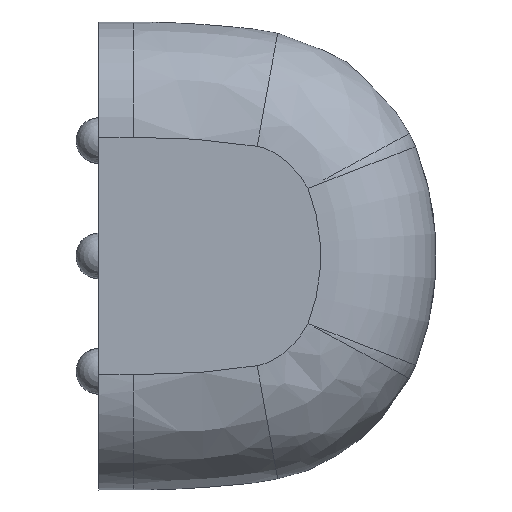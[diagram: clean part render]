
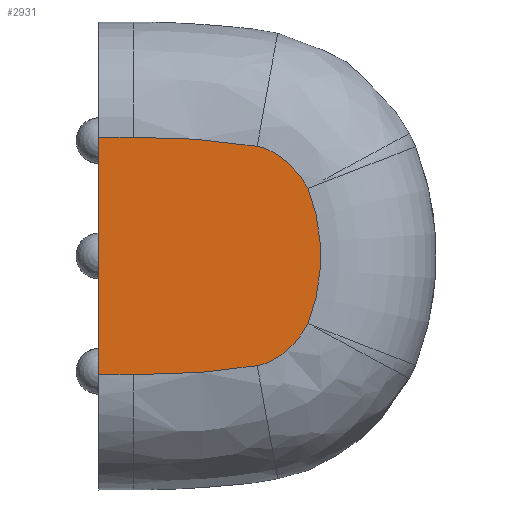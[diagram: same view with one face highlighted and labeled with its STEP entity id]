
A CAD part, front view. The second image highlights one B-rep face of the part: STEP entity #2931.
In plain terms, the highlighted planar face has unit normal (0, -1, 0).
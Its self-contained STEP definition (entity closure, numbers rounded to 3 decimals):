
#60 = PLANE ( 'NONE',  #2061 ) ;
#94 = LINE ( 'NONE', #3117, #1246 ) ;
#139 = ORIENTED_EDGE ( 'NONE', *, *, #1012, .T. ) ;
#150 = CARTESIAN_POINT ( 'NONE',  ( -197.151, -79.943, -4.872 ) ) ;
#158 = CARTESIAN_POINT ( 'NONE',  ( -194.189, -79.943, 11.849 ) ) ;
#170 = VECTOR ( 'NONE', #3133, 1000. ) ;
#292 = ORIENTED_EDGE ( 'NONE', *, *, #4550, .T. ) ;
#363 = EDGE_CURVE ( 'NONE', #2979, #3120, #4912, .T. ) ;
#495 = VERTEX_POINT ( 'NONE', #5963 ) ;
#546 = B_SPLINE_CURVE_WITH_KNOTS ( 'NONE', 3,
 ( #2611, #150, #666, #4102, #1153, #4589, #1658, #5085, #2151, #5576, #2631, #6057 ),
 .UNSPECIFIED., .F., .F.,
 ( 4, 2, 2, 2, 2, 4 ),
 ( 0., 0.001, 0.002, 0.003, 0.004, 0.006 ),
 .UNSPECIFIED. ) ;
#556 = CARTESIAN_POINT ( 'NONE',  ( -193.644, -79.943, -21.728 ) ) ;
#651 = CARTESIAN_POINT ( 'NONE',  ( -194.688, -79.943, 12.395 ) ) ;
#666 = CARTESIAN_POINT ( 'NONE',  ( -196.694, -79.943, -4.699 ) ) ;
#692 = EDGE_CURVE ( 'NONE', #1671, #495, #546, .T. ) ;
#695 = CARTESIAN_POINT ( 'NONE',  ( -201.21, -79.943, 14.543 ) ) ;
#735 = ORIENTED_EDGE ( 'NONE', *, *, #5508, .T. ) ;
#886 = CARTESIAN_POINT ( 'NONE',  ( -202.107, -79.943, -5.524 ) ) ;
#904 = VERTEX_POINT ( 'NONE', #3021 ) ;
#1001 = FACE_OUTER_BOUND ( 'NONE', #3509, .T. ) ;
#1012 = EDGE_CURVE ( 'NONE', #904, #1671, #2285, .T. ) ;
#1022 = AXIS2_PLACEMENT_3D ( 'NONE', #2161, #5590, #2644 ) ;
#1037 = DIRECTION ( 'NONE',  ( 0., 0., -1. ) ) ;
#1045 = DIRECTION ( 'NONE',  ( 0., 1., 0. ) ) ;
#1140 = CARTESIAN_POINT ( 'NONE',  ( -195.233, -79.943, 12.886 ) ) ;
#1153 = CARTESIAN_POINT ( 'NONE',  ( -195.832, -79.943, -4.226 ) ) ;
#1186 = CARTESIAN_POINT ( 'NONE',  ( -204.803, -79.943, 14.792 ) ) ;
#1246 = VECTOR ( 'NONE', #5556, 1000. ) ;
#1385 = CARTESIAN_POINT ( 'NONE',  ( -199.42, -79.943, -5.248 ) ) ;
#1530 = ORIENTED_EDGE ( 'NONE', *, *, #2436, .T. ) ;
#1644 = CARTESIAN_POINT ( 'NONE',  ( -195.828, -79.943, 13.318 ) ) ;
#1658 = CARTESIAN_POINT ( 'NONE',  ( -195.233, -79.943, -3.792 ) ) ;
#1671 = VERTEX_POINT ( 'NONE', #2897 ) ;
#1691 = CARTESIAN_POINT ( 'NONE',  ( -208.404, -79.943, 14.84 ) ) ;
#1882 = CARTESIAN_POINT ( 'NONE',  ( -197.642, -79.943, -4.962 ) ) ;
#1894 = CARTESIAN_POINT ( 'NONE',  ( -211.361, -79.943, -5.745 ) ) ;
#1913 = VERTEX_POINT ( 'NONE', #3108 ) ;
#1935 = EDGE_CURVE ( 'NONE', #4281, #904, #2935, .T. ) ;
#2061 = AXIS2_PLACEMENT_3D ( 'NONE', #556, #1045, #4484 ) ;
#2136 = CARTESIAN_POINT ( 'NONE',  ( -196.694, -79.943, 13.794 ) ) ;
#2151 = CARTESIAN_POINT ( 'NONE',  ( -194.346, -79.943, -2.954 ) ) ;
#2161 = CARTESIAN_POINT ( 'NONE',  ( -208.404, -79.943, 4.547 ) ) ;
#2285 = B_SPLINE_CURVE_WITH_KNOTS ( 'NONE', 3,
 ( #2358, #5292, #3830, #886, #4326, #1385, #4818, #1882 ),
 .UNSPECIFIED., .F., .F.,
 ( 4, 2, 2, 4 ),
 ( 0., 0.005, 0.008, 0.011 ),
 .UNSPECIFIED. ) ;
#2358 = CARTESIAN_POINT ( 'NONE',  ( -208.403, -79.943, -5.745 ) ) ;
#2436 = EDGE_CURVE ( 'NONE', #5596, #1913, #94, .T. ) ;
#2483 = CARTESIAN_POINT ( 'NONE',  ( -211.361, -79.943, -21.728 ) ) ;
#2600 = CARTESIAN_POINT ( 'NONE',  ( -193.466, -79.943, 10.854 ) ) ;
#2611 = CARTESIAN_POINT ( 'NONE',  ( -197.642, -79.943, -4.962 ) ) ;
#2619 = CARTESIAN_POINT ( 'NONE',  ( -197.642, -79.943, 14.056 ) ) ;
#2631 = CARTESIAN_POINT ( 'NONE',  ( -193.466, -79.943, -1.759 ) ) ;
#2642 = CARTESIAN_POINT ( 'NONE',  ( -197.642, -79.943, 14.056 ) ) ;
#2644 = DIRECTION ( 'NONE',  ( -1., 0., 0. ) ) ;
#2897 = CARTESIAN_POINT ( 'NONE',  ( -197.642, -79.943, -4.962 ) ) ;
#2931 = ADVANCED_FACE ( 'NONE', ( #1001 ), #60, .F. ) ;
#2935 = LINE ( 'NONE', #5571, #170 ) ;
#2979 = VERTEX_POINT ( 'NONE', #4503 ) ;
#3021 = CARTESIAN_POINT ( 'NONE',  ( -208.403, -79.943, -5.745 ) ) ;
#3108 = CARTESIAN_POINT ( 'NONE',  ( -211.361, -79.943, 14.84 ) ) ;
#3117 = CARTESIAN_POINT ( 'NONE',  ( -193.644, -79.943, 14.84 ) ) ;
#3120 = VERTEX_POINT ( 'NONE', #4561 ) ;
#3133 = DIRECTION ( 'NONE',  ( 1., 0., 0. ) ) ;
#3509 = EDGE_LOOP ( 'NONE', ( #1530, #735, #3752, #139, #5740, #292, #4438, #4811 ) ) ;
#3585 = CIRCLE ( 'NONE', #1022, 16.269 ) ;
#3605 = CARTESIAN_POINT ( 'NONE',  ( -194.35, -79.943, 12.037 ) ) ;
#3642 = CARTESIAN_POINT ( 'NONE',  ( -199.42, -79.943, 14.342 ) ) ;
#3752 = ORIENTED_EDGE ( 'NONE', *, *, #1935, .T. ) ;
#3830 = CARTESIAN_POINT ( 'NONE',  ( -204.803, -79.943, -5.697 ) ) ;
#4090 = CARTESIAN_POINT ( 'NONE',  ( -194.864, -79.943, 12.565 ) ) ;
#4102 = CARTESIAN_POINT ( 'NONE',  ( -196.044, -79.943, -4.356 ) ) ;
#4134 = CARTESIAN_POINT ( 'NONE',  ( -202.107, -79.943, 14.618 ) ) ;
#4189 = VECTOR ( 'NONE', #1037, 1000. ) ;
#4281 = VERTEX_POINT ( 'NONE', #1894 ) ;
#4326 = CARTESIAN_POINT ( 'NONE',  ( -201.21, -79.943, -5.448 ) ) ;
#4343 = LINE ( 'NONE', #2483, #4189 ) ;
#4438 = ORIENTED_EDGE ( 'NONE', *, *, #363, .T. ) ;
#4484 = DIRECTION ( 'NONE',  ( -1., 0., 0. ) ) ;
#4503 = CARTESIAN_POINT ( 'NONE',  ( -193.231, -79.943, 10.419 ) ) ;
#4550 = EDGE_CURVE ( 'NONE', #495, #2979, #3585, .T. ) ;
#4561 = CARTESIAN_POINT ( 'NONE',  ( -197.642, -79.943, 14.056 ) ) ;
#4575 = CARTESIAN_POINT ( 'NONE',  ( -195.425, -79.943, 13.037 ) ) ;
#4589 = CARTESIAN_POINT ( 'NONE',  ( -195.426, -79.943, -3.943 ) ) ;
#4614 = CARTESIAN_POINT ( 'NONE',  ( -206.602, -79.943, 14.84 ) ) ;
#4811 = ORIENTED_EDGE ( 'NONE', *, *, #6062, .T. ) ;
#4818 = CARTESIAN_POINT ( 'NONE',  ( -198.529, -79.943, -5.123 ) ) ;
#4912 = B_SPLINE_CURVE_WITH_KNOTS ( 'NONE', 3,
 ( #6027, #2600, #5539, #158, #3605, #651, #4090, #1140, #4575, #1644, #5073, #2136, #5560, #2619 ),
 .UNSPECIFIED., .F., .F.,
 ( 4, 2, 2, 2, 2, 2, 4 ),
 ( 0., 0.001, 0.002, 0.003, 0.004, 0.004, 0.006 ),
 .UNSPECIFIED. ) ;
#5073 = CARTESIAN_POINT ( 'NONE',  ( -196.04, -79.943, 13.449 ) ) ;
#5085 = CARTESIAN_POINT ( 'NONE',  ( -194.68, -79.943, -3.31 ) ) ;
#5292 = CARTESIAN_POINT ( 'NONE',  ( -206.603, -79.943, -5.745 ) ) ;
#5508 = EDGE_CURVE ( 'NONE', #1913, #4281, #4343, .T. ) ;
#5539 = CARTESIAN_POINT ( 'NONE',  ( -193.734, -79.943, 11.266 ) ) ;
#5556 = DIRECTION ( 'NONE',  ( -1., 0., 0. ) ) ;
#5560 = CARTESIAN_POINT ( 'NONE',  ( -197.151, -79.943, 13.967 ) ) ;
#5571 = CARTESIAN_POINT ( 'NONE',  ( -193.644, -79.943, -5.745 ) ) ;
#5576 = CARTESIAN_POINT ( 'NONE',  ( -193.737, -79.943, -2.176 ) ) ;
#5590 = DIRECTION ( 'NONE',  ( 0., -1., 0. ) ) ;
#5596 = VERTEX_POINT ( 'NONE', #5952 ) ;
#5628 = B_SPLINE_CURVE_WITH_KNOTS ( 'NONE', 3,
 ( #2642, #6066, #3642, #695, #4134, #1186, #4614, #1691 ),
 .UNSPECIFIED., .F., .F.,
 ( 4, 2, 2, 4 ),
 ( 0., 0.003, 0.005, 0.011 ),
 .UNSPECIFIED. ) ;
#5740 = ORIENTED_EDGE ( 'NONE', *, *, #692, .T. ) ;
#5952 = CARTESIAN_POINT ( 'NONE',  ( -208.404, -79.943, 14.84 ) ) ;
#5963 = CARTESIAN_POINT ( 'NONE',  ( -193.231, -79.943, -1.324 ) ) ;
#6027 = CARTESIAN_POINT ( 'NONE',  ( -193.231, -79.943, 10.419 ) ) ;
#6057 = CARTESIAN_POINT ( 'NONE',  ( -193.231, -79.943, -1.324 ) ) ;
#6062 = EDGE_CURVE ( 'NONE', #3120, #5596, #5628, .T. ) ;
#6066 = CARTESIAN_POINT ( 'NONE',  ( -198.528, -79.943, 14.217 ) ) ;
